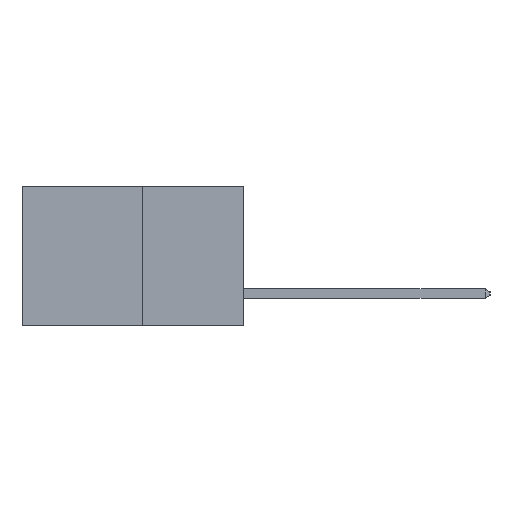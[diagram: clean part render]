
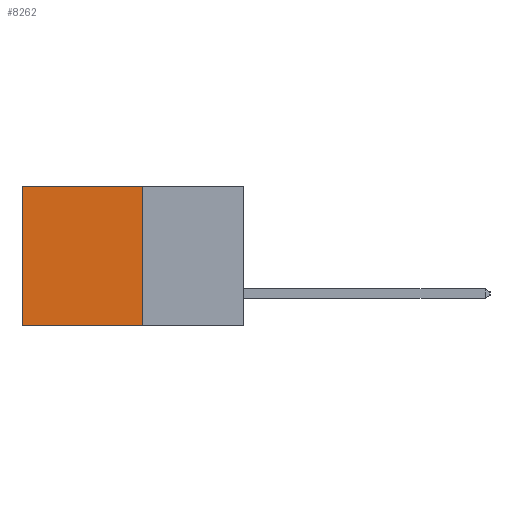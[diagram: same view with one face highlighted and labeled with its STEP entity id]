
A CAD part, left-side view. The second image highlights one B-rep face of the part: STEP entity #8262.
In plain terms, the highlighted planar face has unit normal (-1, 0, 0).
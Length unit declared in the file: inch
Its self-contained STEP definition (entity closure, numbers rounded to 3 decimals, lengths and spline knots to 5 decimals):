
#39 = LINE ( 'NONE', #9122, #4488 ) ;
#230 = VERTEX_POINT ( 'NONE', #11193 ) ;
#233 = CARTESIAN_POINT ( 'NONE',  ( 0.277, 0.59, 0. ) ) ;
#1096 = VERTEX_POINT ( 'NONE', #11242 ) ;
#1320 = PLANE ( 'NONE',  #4235 ) ;
#1663 = DIRECTION ( 'NONE',  ( 0., 0., -1. ) ) ;
#1665 = VERTEX_POINT ( 'NONE', #6527 ) ;
#1702 = CARTESIAN_POINT ( 'NONE',  ( 0.277, 0.27, -0.37 ) ) ;
#2167 = VECTOR ( 'NONE', #1663, 39.37008 ) ;
#2263 = VECTOR ( 'NONE', #7570, 39.37008 ) ;
#2436 = EDGE_CURVE ( 'NONE', #230, #1096, #39, .T. ) ;
#2648 = ORIENTED_EDGE ( 'NONE', *, *, #6254, .F. ) ;
#3181 = VECTOR ( 'NONE', #3347, 39.37008 ) ;
#3238 = CARTESIAN_POINT ( 'NONE',  ( 0.277, 0.59, -0.37 ) ) ;
#3347 = DIRECTION ( 'NONE',  ( 0., 0., -1. ) ) ;
#3780 = ORIENTED_EDGE ( 'NONE', *, *, #2436, .F. ) ;
#4166 = DIRECTION ( 'NONE',  ( 1., 0., 0. ) ) ;
#4235 = AXIS2_PLACEMENT_3D ( 'NONE', #9349, #4166, #10207 ) ;
#4488 = VECTOR ( 'NONE', #10083, 39.37008 ) ;
#4536 = LINE ( 'NONE', #1702, #2167 ) ;
#5936 = EDGE_CURVE ( 'NONE', #9277, #1096, #8108, .T. ) ;
#6254 = EDGE_CURVE ( 'NONE', #1665, #230, #4536, .T. ) ;
#6527 = CARTESIAN_POINT ( 'NONE',  ( 0.277, 0.27, 0. ) ) ;
#6678 = FACE_OUTER_BOUND ( 'NONE', #8438, .T. ) ;
#6984 = EDGE_CURVE ( 'NONE', #1665, #9277, #9232, .T. ) ;
#7559 = ORIENTED_EDGE ( 'NONE', *, *, #5936, .T. ) ;
#7570 = DIRECTION ( 'NONE',  ( 0., 1., 0. ) ) ;
#8108 = LINE ( 'NONE', #3238, #3181 ) ;
#8262 = ADVANCED_FACE ( 'NONE', ( #6678 ), #1320, .F. ) ;
#8438 = EDGE_LOOP ( 'NONE', ( #7559, #3780, #2648, #10301 ) ) ;
#9122 = CARTESIAN_POINT ( 'NONE',  ( 0.277, 0.27, -0.37 ) ) ;
#9232 = LINE ( 'NONE', #10958, #2263 ) ;
#9277 = VERTEX_POINT ( 'NONE', #233 ) ;
#9349 = CARTESIAN_POINT ( 'NONE',  ( 0.277, 0.27, -0.37 ) ) ;
#10083 = DIRECTION ( 'NONE',  ( 0., 1., 0. ) ) ;
#10207 = DIRECTION ( 'NONE',  ( 0., 0., -1. ) ) ;
#10301 = ORIENTED_EDGE ( 'NONE', *, *, #6984, .T. ) ;
#10958 = CARTESIAN_POINT ( 'NONE',  ( 0.277, 0.27, 0. ) ) ;
#11193 = CARTESIAN_POINT ( 'NONE',  ( 0.277, 0.27, -0.37 ) ) ;
#11242 = CARTESIAN_POINT ( 'NONE',  ( 0.277, 0.59, -0.37 ) ) ;
